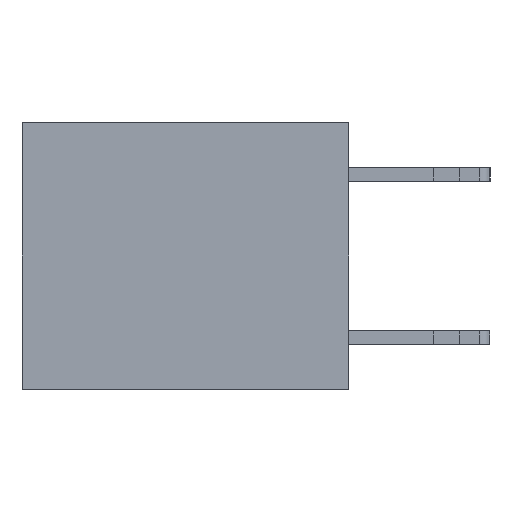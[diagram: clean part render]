
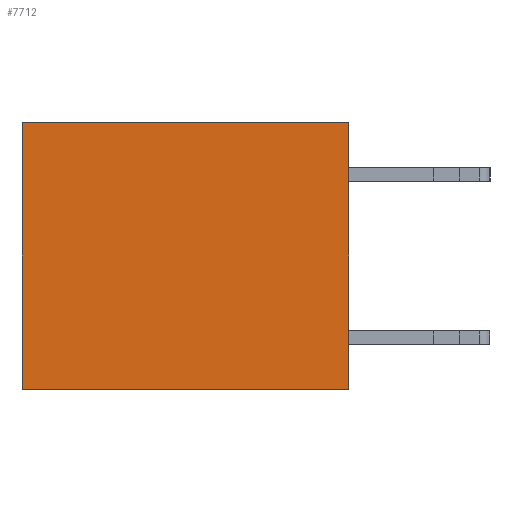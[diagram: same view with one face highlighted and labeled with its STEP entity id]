
A CAD part, left-side view. The second image highlights one B-rep face of the part: STEP entity #7712.
In plain terms, the highlighted planar face has unit normal (-1, 0, 0).
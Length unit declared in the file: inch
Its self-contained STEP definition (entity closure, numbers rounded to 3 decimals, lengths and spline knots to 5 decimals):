
#118 = VERTEX_POINT ( 'NONE', #5261 ) ;
#1120 = LINE ( 'NONE', #10434, #17514 ) ;
#1297 = LINE ( 'NONE', #3879, #1809 ) ;
#1422 = DIRECTION ( 'NONE',  ( 0., 0., -1. ) ) ;
#1809 = VECTOR ( 'NONE', #15003, 39.37008 ) ;
#2354 = LINE ( 'NONE', #3651, #10762 ) ;
#2431 = DIRECTION ( 'NONE',  ( 0., 1., 0. ) ) ;
#3651 = CARTESIAN_POINT ( 'NONE',  ( 0.3165, 0., -0.49 ) ) ;
#3879 = CARTESIAN_POINT ( 'NONE',  ( 0.3165, 0.6, -0.49 ) ) ;
#5261 = CARTESIAN_POINT ( 'NONE',  ( 0.3165, 0., -0.49 ) ) ;
#5767 = EDGE_CURVE ( 'NONE', #11125, #118, #2354, .T. ) ;
#6699 = EDGE_CURVE ( 'NONE', #13554, #12283, #1297, .T. ) ;
#6845 = ORIENTED_EDGE ( 'NONE', *, *, #5767, .F. ) ;
#7562 = CARTESIAN_POINT ( 'NONE',  ( 0.3165, 0., -0.49 ) ) ;
#7712 = ADVANCED_FACE ( 'NONE', ( #14690 ), #10835, .F. ) ;
#7718 = CARTESIAN_POINT ( 'NONE',  ( 0.3165, 0., -0.49 ) ) ;
#8115 = AXIS2_PLACEMENT_3D ( 'NONE', #7718, #10897, #1422 ) ;
#8394 = CARTESIAN_POINT ( 'NONE',  ( 0.3165, 0.6, 0. ) ) ;
#9340 = VECTOR ( 'NONE', #15579, 39.37008 ) ;
#10434 = CARTESIAN_POINT ( 'NONE',  ( 0.3165, 0., 0. ) ) ;
#10762 = VECTOR ( 'NONE', #14785, 39.37008 ) ;
#10835 = PLANE ( 'NONE',  #8115 ) ;
#10897 = DIRECTION ( 'NONE',  ( 1., 0., 0. ) ) ;
#11125 = VERTEX_POINT ( 'NONE', #12293 ) ;
#11246 = EDGE_CURVE ( 'NONE', #11125, #13554, #1120, .T. ) ;
#12283 = VERTEX_POINT ( 'NONE', #15822 ) ;
#12293 = CARTESIAN_POINT ( 'NONE',  ( 0.3165, 0., 0. ) ) ;
#12948 = ORIENTED_EDGE ( 'NONE', *, *, #11246, .T. ) ;
#13554 = VERTEX_POINT ( 'NONE', #8394 ) ;
#13608 = LINE ( 'NONE', #7562, #9340 ) ;
#14690 = FACE_OUTER_BOUND ( 'NONE', #15243, .T. ) ;
#14785 = DIRECTION ( 'NONE',  ( 0., 0., -1. ) ) ;
#15003 = DIRECTION ( 'NONE',  ( 0., 0., -1. ) ) ;
#15243 = EDGE_LOOP ( 'NONE', ( #19452, #19501, #6845, #12948 ) ) ;
#15470 = EDGE_CURVE ( 'NONE', #118, #12283, #13608, .T. ) ;
#15579 = DIRECTION ( 'NONE',  ( 0., 1., 0. ) ) ;
#15822 = CARTESIAN_POINT ( 'NONE',  ( 0.3165, 0.6, -0.49 ) ) ;
#17514 = VECTOR ( 'NONE', #2431, 39.37008 ) ;
#19452 = ORIENTED_EDGE ( 'NONE', *, *, #6699, .T. ) ;
#19501 = ORIENTED_EDGE ( 'NONE', *, *, #15470, .F. ) ;
